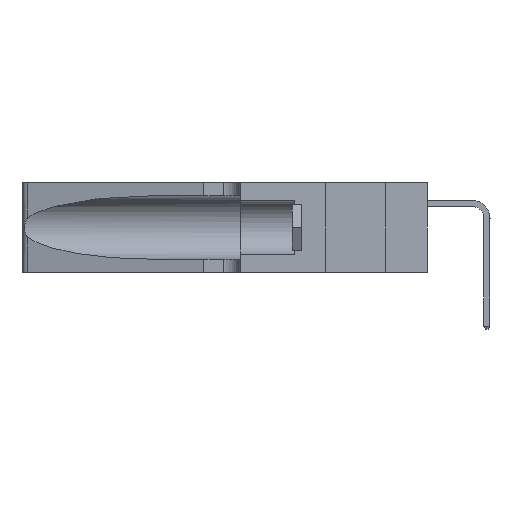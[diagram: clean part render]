
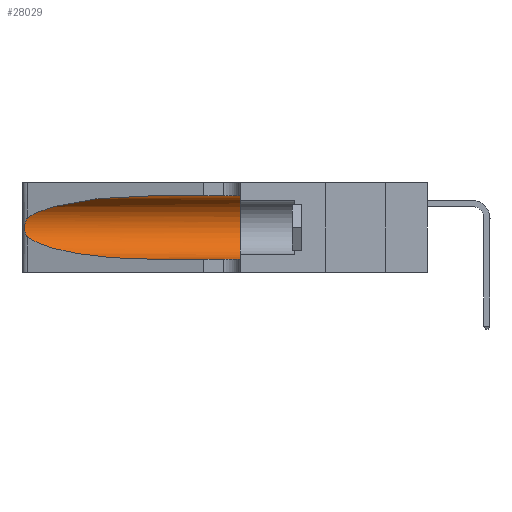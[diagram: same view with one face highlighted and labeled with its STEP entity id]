
A CAD part, left-side view. The second image highlights one B-rep face of the part: STEP entity #28029.
In plain terms, the highlighted cylindrical face has radius 3.308 mm (diameter 6.617 mm), a partial arc.
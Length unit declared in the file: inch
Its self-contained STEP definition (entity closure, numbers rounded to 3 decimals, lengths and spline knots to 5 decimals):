
#737 = VERTEX_POINT ( 'NONE', #17597 ) ;
#837 =( BOUNDED_CURVE ( )  B_SPLINE_CURVE ( 3, ( #5761, #9334, #16573, #41548 ),
 .UNSPECIFIED., .F., .F. ) 
 B_SPLINE_CURVE_WITH_KNOTS ( ( 4, 4 ),
 ( 3.44316, 4.71239 ),
 .UNSPECIFIED. ) 
 CURVE ( )  GEOMETRIC_REPRESENTATION_ITEM ( )  RATIONAL_B_SPLINE_CURVE ( ( 1., 0.87, 0.87, 1. ) ) 
 REPRESENTATION_ITEM ( '' )  );
#1299 = ORIENTED_EDGE ( 'NONE', *, *, #8882, .T. ) ;
#1896 = VERTEX_POINT ( 'NONE', #40003 ) ;
#1937 = VECTOR ( 'NONE', #45047, 39.37008 ) ;
#2175 = CARTESIAN_POINT ( 'NONE',  ( 0.1305, 1.61858, 0.31525 ) ) ;
#3017 = CARTESIAN_POINT ( 'NONE',  ( 0.25787, 1.23484, 0.2124 ) ) ;
#3060 = LINE ( 'NONE', #2175, #1937 ) ;
#3398 = ORIENTED_EDGE ( 'NONE', *, *, #4019, .T. ) ;
#3414 = DIRECTION ( 'NONE',  ( 0., 1., 0. ) ) ;
#3844 = CYLINDRICAL_SURFACE ( 'NONE', #6230, 0.13025 ) ;
#4019 = EDGE_CURVE ( 'NONE', #45950, #36633, #19782, .T. ) ;
#5761 = CARTESIAN_POINT ( 'NONE',  ( 0.25487, 1.22718, 0.14631 ) ) ;
#6230 = AXIS2_PLACEMENT_3D ( 'NONE', #23612, #27208, #19997 ) ;
#6601 = CARTESIAN_POINT ( 'NONE',  ( 0.26018, 1.23835, 0.19895 ) ) ;
#7255 = CARTESIAN_POINT ( 'NONE',  ( 0.1305, 1.61858, 0.05475 ) ) ;
#7744 = ORIENTED_EDGE ( 'NONE', *, *, #43107, .F. ) ;
#8381 = CARTESIAN_POINT ( 'NONE',  ( 0.18966, 0.96281, 0.31525 ) ) ;
#8882 = EDGE_CURVE ( 'NONE', #11864, #1896, #42414, .T. ) ;
#9334 = CARTESIAN_POINT ( 'NONE',  ( 0.2373, 1.15595, 0.08982 ) ) ;
#10093 = VERTEX_POINT ( 'NONE', #15166 ) ;
#10179 = CARTESIAN_POINT ( 'NONE',  ( 0.26075, 1.23896, 0.178 ) ) ;
#10835 = DIRECTION ( 'NONE',  ( 0., -1., 0. ) ) ;
#10969 = ORIENTED_EDGE ( 'NONE', *, *, #36080, .T. ) ;
#11461 = EDGE_LOOP ( 'NONE', ( #1299, #10969, #44316, #3398, #7744, #30800 ) ) ;
#11864 = VERTEX_POINT ( 'NONE', #27632 ) ;
#13133 = CARTESIAN_POINT ( 'NONE',  ( 0.1305, 0.35, 0.05475 ) ) ;
#13814 = CARTESIAN_POINT ( 'NONE',  ( 0.25856, 1.23593, 0.16098 ) ) ;
#14036 = B_SPLINE_CURVE_WITH_KNOTS ( 'NONE', 3,
 ( #20853, #17233, #24486, #3017, #28047, #6601, #31626, #10179, #35240, #13814, #38804, #17401, #42408, #21032 ),
 .UNSPECIFIED., .F., .F.,
 ( 4, 2, 2, 2, 2, 2, 4 ),
 ( 0., 0.00027, 0.00053, 0.00107, 0.0016, 0.00187, 0.00214 ),
 .UNSPECIFIED. ) ;
#15166 = CARTESIAN_POINT ( 'NONE',  ( 0.1305, 0.35, 0.31525 ) ) ;
#15596 = CARTESIAN_POINT ( 'NONE',  ( 0.2373, 1.15595, 0.28018 ) ) ;
#16573 = CARTESIAN_POINT ( 'NONE',  ( 0.18966, 0.96281, 0.05475 ) ) ;
#17233 = CARTESIAN_POINT ( 'NONE',  ( 0.25555, 1.22994, 0.2215 ) ) ;
#17401 = CARTESIAN_POINT ( 'NONE',  ( 0.25639, 1.23186, 0.15144 ) ) ;
#17597 = CARTESIAN_POINT ( 'NONE',  ( 0.25487, 1.22718, 0.14631 ) ) ;
#19782 = LINE ( 'NONE', #7255, #28171 ) ;
#19997 = DIRECTION ( 'NONE',  ( 0., 0., -1. ) ) ;
#20853 = CARTESIAN_POINT ( 'NONE',  ( 0.25487, 1.22718, 0.22369 ) ) ;
#21032 = CARTESIAN_POINT ( 'NONE',  ( 0.25487, 1.22718, 0.14631 ) ) ;
#23612 = CARTESIAN_POINT ( 'NONE',  ( 0.1305, 1.61858, 0.185 ) ) ;
#24432 = EDGE_CURVE ( 'NONE', #737, #45950, #837, .T. ) ;
#24486 = CARTESIAN_POINT ( 'NONE',  ( 0.25639, 1.23184, 0.21858 ) ) ;
#24910 = CARTESIAN_POINT ( 'NONE',  ( 0.1305, 0.35, 0.185 ) ) ;
#27208 = DIRECTION ( 'NONE',  ( 0., -1., 0. ) ) ;
#27632 = CARTESIAN_POINT ( 'NONE',  ( 0.1305, 0.72297, 0.31525 ) ) ;
#27829 = AXIS2_PLACEMENT_3D ( 'NONE', #24910, #3414, #28455 ) ;
#28029 = ADVANCED_FACE ( 'NONE', ( #32393 ), #3844, .F. ) ;
#28047 = CARTESIAN_POINT ( 'NONE',  ( 0.25854, 1.2359, 0.20912 ) ) ;
#28171 = VECTOR ( 'NONE', #10835, 39.37008 ) ;
#28455 = DIRECTION ( 'NONE',  ( 0., 0., 1. ) ) ;
#30800 = ORIENTED_EDGE ( 'NONE', *, *, #31099, .F. ) ;
#31099 = EDGE_CURVE ( 'NONE', #11864, #10093, #3060, .T. ) ;
#31626 = CARTESIAN_POINT ( 'NONE',  ( 0.26075, 1.23896, 0.19203 ) ) ;
#32393 = FACE_OUTER_BOUND ( 'NONE', #11461, .T. ) ;
#33435 = CARTESIAN_POINT ( 'NONE',  ( 0.1305, 0.72297, 0.31525 ) ) ;
#35240 = CARTESIAN_POINT ( 'NONE',  ( 0.26017, 1.23833, 0.17102 ) ) ;
#36080 = EDGE_CURVE ( 'NONE', #1896, #737, #14036, .T. ) ;
#36633 = VERTEX_POINT ( 'NONE', #13133 ) ;
#38804 = CARTESIAN_POINT ( 'NONE',  ( 0.25789, 1.23486, 0.15765 ) ) ;
#40003 = CARTESIAN_POINT ( 'NONE',  ( 0.25487, 1.22718, 0.22369 ) ) ;
#40591 = CARTESIAN_POINT ( 'NONE',  ( 0.25487, 1.22718, 0.22369 ) ) ;
#41548 = CARTESIAN_POINT ( 'NONE',  ( 0.1305, 0.72297, 0.05475 ) ) ;
#41850 = CIRCLE ( 'NONE', #27829, 0.13025 ) ;
#42408 = CARTESIAN_POINT ( 'NONE',  ( 0.25555, 1.22993, 0.14849 ) ) ;
#42414 =( BOUNDED_CURVE ( )  B_SPLINE_CURVE ( 3, ( #33435, #8381, #15596, #40591 ),
 .UNSPECIFIED., .F., .T. ) 
 B_SPLINE_CURVE_WITH_KNOTS ( ( 4, 4 ),
 ( 1.5708, 2.84003 ),
 .UNSPECIFIED. ) 
 CURVE ( )  GEOMETRIC_REPRESENTATION_ITEM ( )  RATIONAL_B_SPLINE_CURVE ( ( 1., 0.87, 0.87, 1. ) ) 
 REPRESENTATION_ITEM ( '' )  );
#43107 = EDGE_CURVE ( 'NONE', #10093, #36633, #41850, .T. ) ;
#44316 = ORIENTED_EDGE ( 'NONE', *, *, #24432, .T. ) ;
#44801 = CARTESIAN_POINT ( 'NONE',  ( 0.1305, 0.72297, 0.05475 ) ) ;
#45047 = DIRECTION ( 'NONE',  ( 0., -1., 0. ) ) ;
#45950 = VERTEX_POINT ( 'NONE', #44801 ) ;
